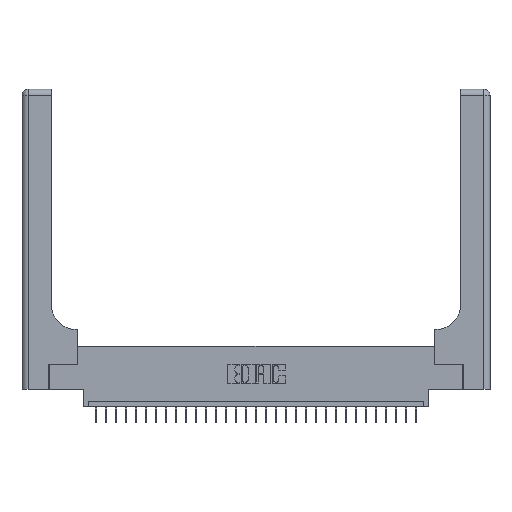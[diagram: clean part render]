
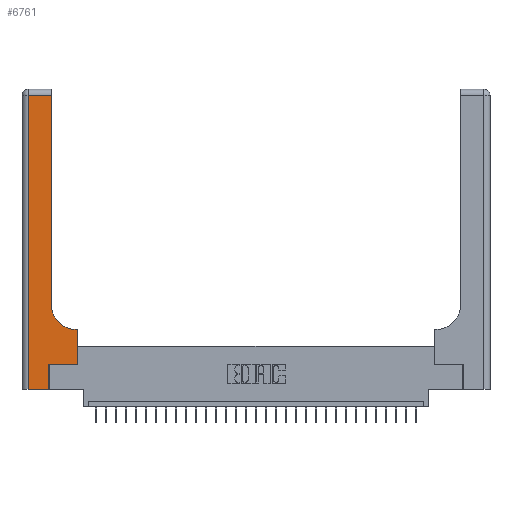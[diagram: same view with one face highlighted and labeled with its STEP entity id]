
A CAD part, top view. The second image highlights one B-rep face of the part: STEP entity #6761.
In plain terms, the highlighted planar face has unit normal (0, 0, 1).
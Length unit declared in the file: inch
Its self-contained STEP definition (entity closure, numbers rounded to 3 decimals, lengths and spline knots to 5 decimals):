
#745 = CARTESIAN_POINT ( 'NONE',  ( 0.2915, 0.6, 0.37 ) ) ;
#1198 = ORIENTED_EDGE ( 'NONE', *, *, #17426, .T. ) ;
#1371 = ORIENTED_EDGE ( 'NONE', *, *, #2755, .T. ) ;
#2593 = EDGE_LOOP ( 'NONE', ( #19297, #28932, #13048, #1198, #26244, #15221, #1371, #14329, #19428 ) ) ;
#2755 = EDGE_CURVE ( 'NONE', #17570, #23108, #23129, .T. ) ;
#3101 = EDGE_CURVE ( 'NONE', #23108, #24424, #26883, .T. ) ;
#3907 = CARTESIAN_POINT ( 'NONE',  ( 0.2915, 0.85, 0.37 ) ) ;
#4072 = VECTOR ( 'NONE', #26131, 39.37008 ) ;
#4369 = FACE_OUTER_BOUND ( 'NONE', #2593, .T. ) ;
#4423 = LINE ( 'NONE', #13924, #4072 ) ;
#4467 = CARTESIAN_POINT ( 'NONE',  ( 0.06, 2.94, 0.37 ) ) ;
#4648 = DIRECTION ( 'NONE',  ( -1., 0., 0. ) ) ;
#4655 = VERTEX_POINT ( 'NONE', #8356 ) ;
#5505 = DIRECTION ( 'NONE',  ( 1., 0., 0. ) ) ;
#5647 = DIRECTION ( 'NONE',  ( -1., 0., 0. ) ) ;
#5678 = EDGE_CURVE ( 'NONE', #6404, #4655, #4423, .T. ) ;
#6332 = DIRECTION ( 'NONE',  ( 0., 0., -1. ) ) ;
#6404 = VERTEX_POINT ( 'NONE', #4467 ) ;
#6761 = ADVANCED_FACE ( 'NONE', ( #4369 ), #10916, .F. ) ;
#6826 = EDGE_CURVE ( 'NONE', #17904, #6404, #8890, .T. ) ;
#7108 = CIRCLE ( 'NONE', #15819, 0.25 ) ;
#7266 = LINE ( 'NONE', #15214, #22563 ) ;
#7534 = EDGE_CURVE ( 'NONE', #23374, #17904, #29712, .T. ) ;
#7644 = VECTOR ( 'NONE', #11166, 39.37008 ) ;
#8356 = CARTESIAN_POINT ( 'NONE',  ( 0.06, 0., 0.37 ) ) ;
#8667 = EDGE_CURVE ( 'NONE', #15665, #13951, #11067, .T. ) ;
#8890 = LINE ( 'NONE', #19183, #29769 ) ;
#10306 = EDGE_CURVE ( 'NONE', #13951, #17570, #7266, .T. ) ;
#10491 = DIRECTION ( 'NONE',  ( 0., 1., 0. ) ) ;
#10743 = VECTOR ( 'NONE', #26715, 39.37008 ) ;
#10916 = PLANE ( 'NONE',  #20652 ) ;
#11044 = DIRECTION ( 'NONE',  ( 1., 0., 0. ) ) ;
#11067 = LINE ( 'NONE', #25685, #7644 ) ;
#11166 = DIRECTION ( 'NONE',  ( 0., 1., 0. ) ) ;
#11196 = VECTOR ( 'NONE', #5505, 39.37008 ) ;
#11325 = CARTESIAN_POINT ( 'NONE',  ( 0.5585, 0.25, 0.37 ) ) ;
#12331 = LINE ( 'NONE', #14942, #11196 ) ;
#13048 = ORIENTED_EDGE ( 'NONE', *, *, #5678, .T. ) ;
#13264 = CARTESIAN_POINT ( 'NONE',  ( 0.5415, 0.6, 0.37 ) ) ;
#13924 = CARTESIAN_POINT ( 'NONE',  ( 0.06, 3., 0.37 ) ) ;
#13951 = VERTEX_POINT ( 'NONE', #23044 ) ;
#14329 = ORIENTED_EDGE ( 'NONE', *, *, #3101, .T. ) ;
#14942 = CARTESIAN_POINT ( 'NONE',  ( 0., 0., 0.37 ) ) ;
#15214 = CARTESIAN_POINT ( 'NONE',  ( 0.269, 0.25, 0.37 ) ) ;
#15221 = ORIENTED_EDGE ( 'NONE', *, *, #10306, .T. ) ;
#15665 = VERTEX_POINT ( 'NONE', #20438 ) ;
#15789 = CARTESIAN_POINT ( 'NONE',  ( 0., 3., 0.37 ) ) ;
#15819 = AXIS2_PLACEMENT_3D ( 'NONE', #16124, #20591, #11044 ) ;
#16124 = CARTESIAN_POINT ( 'NONE',  ( 0.5415, 0.85, 0.37 ) ) ;
#16279 = VECTOR ( 'NONE', #5647, 39.37008 ) ;
#17173 = CARTESIAN_POINT ( 'NONE',  ( 0.2915, 3., 0.37 ) ) ;
#17426 = EDGE_CURVE ( 'NONE', #4655, #15665, #12331, .T. ) ;
#17495 = CARTESIAN_POINT ( 'NONE',  ( 0.5585, 0.25, 0.37 ) ) ;
#17570 = VERTEX_POINT ( 'NONE', #11325 ) ;
#17904 = VERTEX_POINT ( 'NONE', #20456 ) ;
#19183 = CARTESIAN_POINT ( 'NONE',  ( 0., 2.94, 0.37 ) ) ;
#19297 = ORIENTED_EDGE ( 'NONE', *, *, #7534, .T. ) ;
#19428 = ORIENTED_EDGE ( 'NONE', *, *, #22199, .T. ) ;
#20438 = CARTESIAN_POINT ( 'NONE',  ( 0.269, 0., 0.37 ) ) ;
#20456 = CARTESIAN_POINT ( 'NONE',  ( 0.2915, 2.94, 0.37 ) ) ;
#20591 = DIRECTION ( 'NONE',  ( 0., 0., -1. ) ) ;
#20652 = AXIS2_PLACEMENT_3D ( 'NONE', #15789, #6332, #20668 ) ;
#20668 = DIRECTION ( 'NONE',  ( -1., 0., 0. ) ) ;
#21597 = VECTOR ( 'NONE', #10491, 39.37008 ) ;
#22199 = EDGE_CURVE ( 'NONE', #24424, #23374, #7108, .T. ) ;
#22563 = VECTOR ( 'NONE', #30059, 39.37008 ) ;
#23044 = CARTESIAN_POINT ( 'NONE',  ( 0.269, 0.25, 0.37 ) ) ;
#23108 = VERTEX_POINT ( 'NONE', #26162 ) ;
#23129 = LINE ( 'NONE', #17495, #21597 ) ;
#23374 = VERTEX_POINT ( 'NONE', #3907 ) ;
#24424 = VERTEX_POINT ( 'NONE', #13264 ) ;
#25685 = CARTESIAN_POINT ( 'NONE',  ( 0.269, 0., 0.37 ) ) ;
#26131 = DIRECTION ( 'NONE',  ( 0., -1., 0. ) ) ;
#26162 = CARTESIAN_POINT ( 'NONE',  ( 0.5585, 0.6, 0.37 ) ) ;
#26244 = ORIENTED_EDGE ( 'NONE', *, *, #8667, .T. ) ;
#26715 = DIRECTION ( 'NONE',  ( 0., 1., 0. ) ) ;
#26883 = LINE ( 'NONE', #745, #16279 ) ;
#28932 = ORIENTED_EDGE ( 'NONE', *, *, #6826, .T. ) ;
#29712 = LINE ( 'NONE', #17173, #10743 ) ;
#29769 = VECTOR ( 'NONE', #4648, 39.37008 ) ;
#30059 = DIRECTION ( 'NONE',  ( 1., 0., 0. ) ) ;
